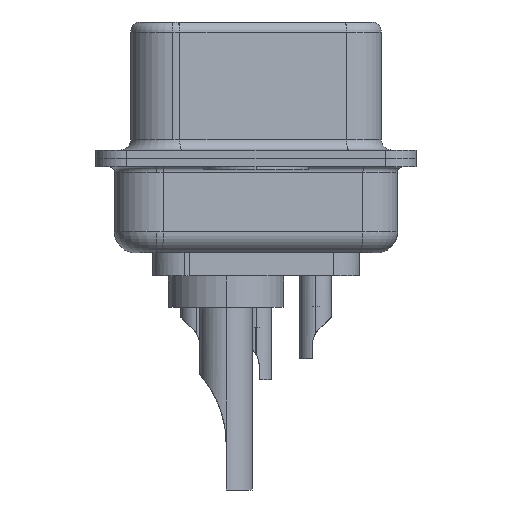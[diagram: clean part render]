
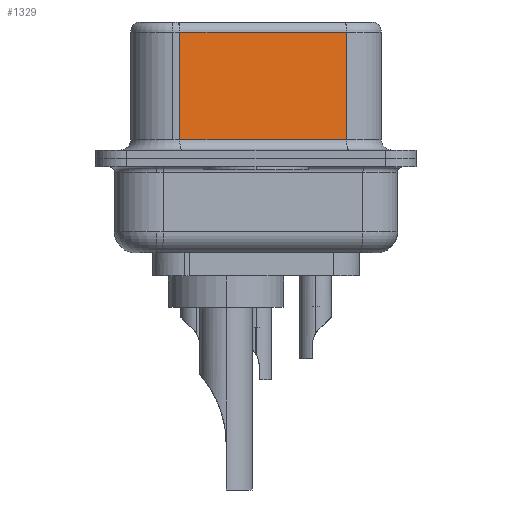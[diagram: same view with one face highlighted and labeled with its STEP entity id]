
A CAD part, left-side view. The second image highlights one B-rep face of the part: STEP entity #1329.
In plain terms, the highlighted planar face has unit normal (-0.985, -0.174, 0).
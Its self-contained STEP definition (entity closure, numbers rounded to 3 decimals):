
#31 = EDGE_CURVE ( 'NONE', #14547, #14508, #16435, .T. ) ;
#762 = ORIENTED_EDGE ( 'NONE', *, *, #11242, .T. ) ;
#1329 = ADVANCED_FACE ( 'NONE', ( #2086 ), #3547, .F. ) ;
#1691 = ORIENTED_EDGE ( 'NONE', *, *, #31, .T. ) ;
#2086 = FACE_OUTER_BOUND ( 'NONE', #8105, .T. ) ;
#3194 = DIRECTION ( 'NONE',  ( -0.174, 0.985, 0. ) ) ;
#3547 = PLANE ( 'NONE',  #10751 ) ;
#4306 = ORIENTED_EDGE ( 'NONE', *, *, #9831, .F. ) ;
#4400 = EDGE_CURVE ( 'NONE', #6531, #13563, #22326, .T. ) ;
#6531 = VERTEX_POINT ( 'NONE', #16303 ) ;
#8105 = EDGE_LOOP ( 'NONE', ( #4306, #1691, #762, #16340 ) ) ;
#9831 = EDGE_CURVE ( 'NONE', #14547, #13563, #23099, .T. ) ;
#10751 = AXIS2_PLACEMENT_3D ( 'NONE', #15899, #20998, #3194 ) ;
#11099 = CARTESIAN_POINT ( 'NONE',  ( 5.132, -4.322, 6.52 ) ) ;
#11228 = VECTOR ( 'NONE', #21943, 1000. ) ;
#11242 = EDGE_CURVE ( 'NONE', #14508, #6531, #17288, .T. ) ;
#11375 = VECTOR ( 'NONE', #23283, 1000. ) ;
#13563 = VERTEX_POINT ( 'NONE', #22966 ) ;
#14249 = CARTESIAN_POINT ( 'NONE',  ( 3.73, 3.628, 6.02 ) ) ;
#14428 = CARTESIAN_POINT ( 'NONE',  ( 5.132, -4.322, 6.02 ) ) ;
#14508 = VERTEX_POINT ( 'NONE', #14249 ) ;
#14547 = VERTEX_POINT ( 'NONE', #14428 ) ;
#15899 = CARTESIAN_POINT ( 'NONE',  ( 5.132, -4.322, 6.52 ) ) ;
#16041 = VECTOR ( 'NONE', #18343, 1000. ) ;
#16303 = CARTESIAN_POINT ( 'NONE',  ( 3.73, 3.628, 0.9 ) ) ;
#16340 = ORIENTED_EDGE ( 'NONE', *, *, #4400, .T. ) ;
#16348 = CARTESIAN_POINT ( 'NONE',  ( 3.73, 3.628, 6.52 ) ) ;
#16362 = CARTESIAN_POINT ( 'NONE',  ( 5.132, -4.322, 6.02 ) ) ;
#16435 = LINE ( 'NONE', #16362, #11228 ) ;
#16610 = CARTESIAN_POINT ( 'NONE',  ( 5.132, -4.322, 0.9 ) ) ;
#17288 = LINE ( 'NONE', #16348, #16041 ) ;
#18343 = DIRECTION ( 'NONE',  ( 0., 0., -1. ) ) ;
#18937 = DIRECTION ( 'NONE',  ( 0., 0., -1. ) ) ;
#19270 = VECTOR ( 'NONE', #18937, 1000. ) ;
#20998 = DIRECTION ( 'NONE',  ( 0.985, 0.174, 0. ) ) ;
#21943 = DIRECTION ( 'NONE',  ( -0.174, 0.985, 0. ) ) ;
#22326 = LINE ( 'NONE', #16610, #11375 ) ;
#22966 = CARTESIAN_POINT ( 'NONE',  ( 5.132, -4.322, 0.9 ) ) ;
#23099 = LINE ( 'NONE', #11099, #19270 ) ;
#23283 = DIRECTION ( 'NONE',  ( 0.174, -0.985, 0. ) ) ;
